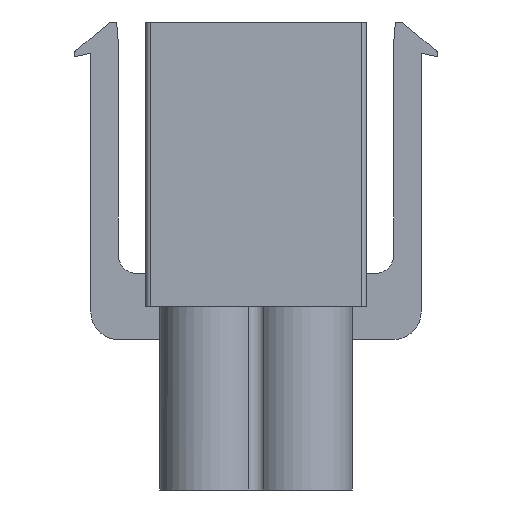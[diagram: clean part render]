
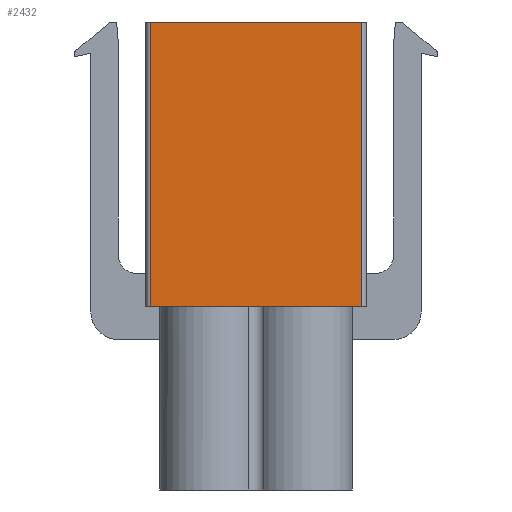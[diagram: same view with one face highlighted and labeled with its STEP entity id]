
A CAD part, front view. The second image highlights one B-rep face of the part: STEP entity #2432.
In plain terms, the highlighted planar face has unit normal (0, -1, 0).
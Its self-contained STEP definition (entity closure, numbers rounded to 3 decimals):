
#995 = DIRECTION ( 'NONE',  ( 0., 0., 1. ) ) ;
#1303 = DIRECTION ( 'NONE',  ( 0., 0., -1. ) ) ;
#1638 = EDGE_CURVE ( 'NONE', #10881, #6717, #5347, .T. ) ;
#1922 = CARTESIAN_POINT ( 'NONE',  ( 5.75, -7., -15.5 ) ) ;
#2097 = PLANE ( 'NONE',  #4354 ) ;
#2195 = CARTESIAN_POINT ( 'NONE',  ( -5.75, -7., -15.5 ) ) ;
#2231 = EDGE_CURVE ( 'NONE', #9150, #8163, #7294, .T. ) ;
#2288 = VECTOR ( 'NONE', #10146, 1000. ) ;
#2432 = ADVANCED_FACE ( 'NONE', ( #5006 ), #2097, .T. ) ;
#2530 = ORIENTED_EDGE ( 'NONE', *, *, #4518, .T. ) ;
#2583 = VECTOR ( 'NONE', #1303, 1000. ) ;
#3026 = DIRECTION ( 'NONE',  ( 0., -1., 0. ) ) ;
#4354 = AXIS2_PLACEMENT_3D ( 'NONE', #7713, #3026, #5878 ) ;
#4518 = EDGE_CURVE ( 'NONE', #6717, #8163, #9513, .T. ) ;
#4568 = VECTOR ( 'NONE', #5447, 1000. ) ;
#4642 = CARTESIAN_POINT ( 'NONE',  ( -6., -7., 0. ) ) ;
#5006 = FACE_OUTER_BOUND ( 'NONE', #9337, .T. ) ;
#5347 = LINE ( 'NONE', #5409, #2288 ) ;
#5409 = CARTESIAN_POINT ( 'NONE',  ( -6., -7., -15.5 ) ) ;
#5447 = DIRECTION ( 'NONE',  ( 1., 0., 0. ) ) ;
#5591 = CARTESIAN_POINT ( 'NONE',  ( 5.75, -7., -15.5 ) ) ;
#5878 = DIRECTION ( 'NONE',  ( 0., 0., -1. ) ) ;
#6717 = VERTEX_POINT ( 'NONE', #5591 ) ;
#6927 = LINE ( 'NONE', #7726, #2583 ) ;
#7294 = LINE ( 'NONE', #4642, #4568 ) ;
#7331 = VECTOR ( 'NONE', #995, 1000. ) ;
#7429 = ORIENTED_EDGE ( 'NONE', *, *, #1638, .T. ) ;
#7713 = CARTESIAN_POINT ( 'NONE',  ( -6., -7., -15.5 ) ) ;
#7726 = CARTESIAN_POINT ( 'NONE',  ( -5.75, -7., -15.5 ) ) ;
#8163 = VERTEX_POINT ( 'NONE', #11058 ) ;
#8509 = ORIENTED_EDGE ( 'NONE', *, *, #2231, .F. ) ;
#9150 = VERTEX_POINT ( 'NONE', #10608 ) ;
#9337 = EDGE_LOOP ( 'NONE', ( #8509, #11617, #7429, #2530 ) ) ;
#9513 = LINE ( 'NONE', #1922, #7331 ) ;
#10146 = DIRECTION ( 'NONE',  ( 1., 0., 0. ) ) ;
#10608 = CARTESIAN_POINT ( 'NONE',  ( -5.75, -7., 0. ) ) ;
#10881 = VERTEX_POINT ( 'NONE', #2195 ) ;
#11058 = CARTESIAN_POINT ( 'NONE',  ( 5.75, -7., 0. ) ) ;
#11539 = EDGE_CURVE ( 'NONE', #9150, #10881, #6927, .T. ) ;
#11617 = ORIENTED_EDGE ( 'NONE', *, *, #11539, .T. ) ;
